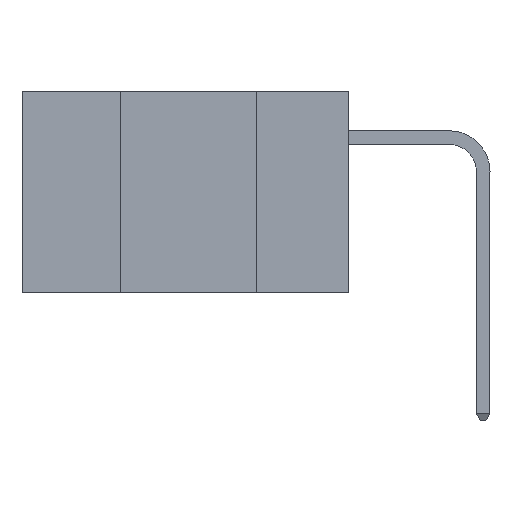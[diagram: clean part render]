
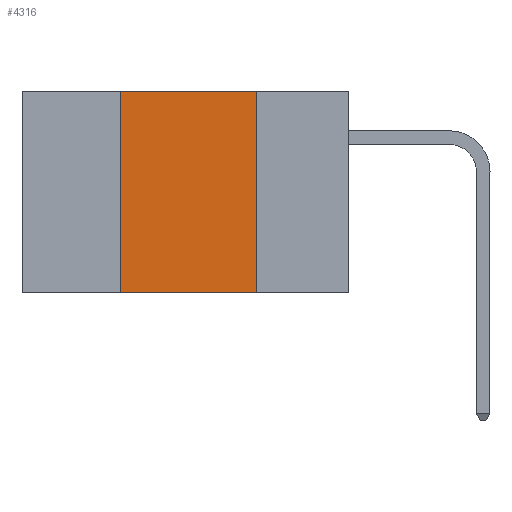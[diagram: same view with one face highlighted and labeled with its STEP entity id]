
A CAD part, left-side view. The second image highlights one B-rep face of the part: STEP entity #4316.
In plain terms, the highlighted planar face has unit normal (-1, 0, 0).
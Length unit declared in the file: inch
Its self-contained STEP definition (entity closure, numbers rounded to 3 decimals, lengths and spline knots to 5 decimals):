
#329 = EDGE_CURVE ( 'NONE', #7540, #8060, #6590, .T. ) ;
#510 = CARTESIAN_POINT ( 'NONE',  ( 0., 0.6, 0. ) ) ;
#718 = CARTESIAN_POINT ( 'NONE',  ( 0., 0.17, 0. ) ) ;
#2082 = VECTOR ( 'NONE', #6203, 39.37008 ) ;
#2097 = VERTEX_POINT ( 'NONE', #5747 ) ;
#2306 = EDGE_CURVE ( 'NONE', #8060, #11072, #3148, .T. ) ;
#2312 = EDGE_CURVE ( 'NONE', #2097, #7540, #3162, .T. ) ;
#2414 = LINE ( 'NONE', #4183, #2082 ) ;
#2425 = EDGE_CURVE ( 'NONE', #2097, #11072, #2414, .T. ) ;
#2568 = CARTESIAN_POINT ( 'NONE',  ( 0., 0.6, 0. ) ) ;
#2784 = PLANE ( 'NONE',  #8957 ) ;
#3102 = VECTOR ( 'NONE', #6044, 39.37008 ) ;
#3148 = LINE ( 'NONE', #718, #3102 ) ;
#3162 = LINE ( 'NONE', #11268, #3440 ) ;
#3440 = VECTOR ( 'NONE', #9247, 39.37008 ) ;
#3875 = DIRECTION ( 'NONE',  ( 0., 0., -1. ) ) ;
#4183 = CARTESIAN_POINT ( 'NONE',  ( 0., 0.6, -0.37 ) ) ;
#4266 = DIRECTION ( 'NONE',  ( 0., -1., 0. ) ) ;
#4316 = ADVANCED_FACE ( 'NONE', ( #8070 ), #2784, .F. ) ;
#5182 = CARTESIAN_POINT ( 'NONE',  ( 0., 0.17, 0. ) ) ;
#5747 = CARTESIAN_POINT ( 'NONE',  ( 0., 0.42, -0.37 ) ) ;
#6044 = DIRECTION ( 'NONE',  ( 0., 0., -1. ) ) ;
#6203 = DIRECTION ( 'NONE',  ( 0., -1., 0. ) ) ;
#6533 = VECTOR ( 'NONE', #4266, 39.37008 ) ;
#6590 = LINE ( 'NONE', #2568, #6533 ) ;
#7473 = ORIENTED_EDGE ( 'NONE', *, *, #2425, .T. ) ;
#7540 = VERTEX_POINT ( 'NONE', #9570 ) ;
#7780 = ORIENTED_EDGE ( 'NONE', *, *, #2312, .F. ) ;
#8060 = VERTEX_POINT ( 'NONE', #5182 ) ;
#8070 = FACE_OUTER_BOUND ( 'NONE', #9471, .T. ) ;
#8090 = ORIENTED_EDGE ( 'NONE', *, *, #2306, .F. ) ;
#8901 = CARTESIAN_POINT ( 'NONE',  ( 0., 0.17, -0.37 ) ) ;
#8957 = AXIS2_PLACEMENT_3D ( 'NONE', #510, #9112, #3875 ) ;
#9112 = DIRECTION ( 'NONE',  ( 1., 0., 0. ) ) ;
#9247 = DIRECTION ( 'NONE',  ( 0., 0., 1. ) ) ;
#9471 = EDGE_LOOP ( 'NONE', ( #8090, #10818, #7780, #7473 ) ) ;
#9570 = CARTESIAN_POINT ( 'NONE',  ( 0., 0.42, 0. ) ) ;
#10818 = ORIENTED_EDGE ( 'NONE', *, *, #329, .F. ) ;
#11072 = VERTEX_POINT ( 'NONE', #8901 ) ;
#11268 = CARTESIAN_POINT ( 'NONE',  ( 0., 0.42, 0. ) ) ;
